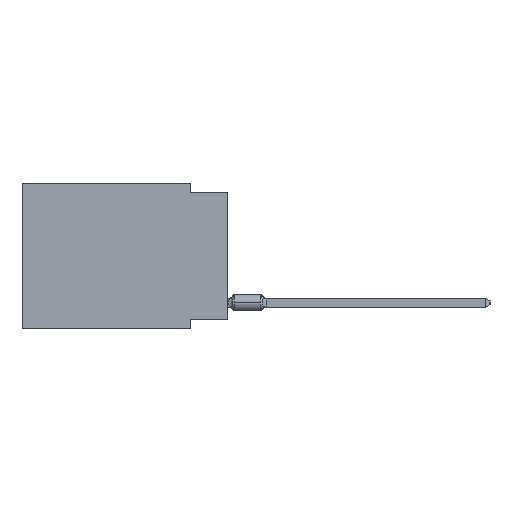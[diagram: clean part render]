
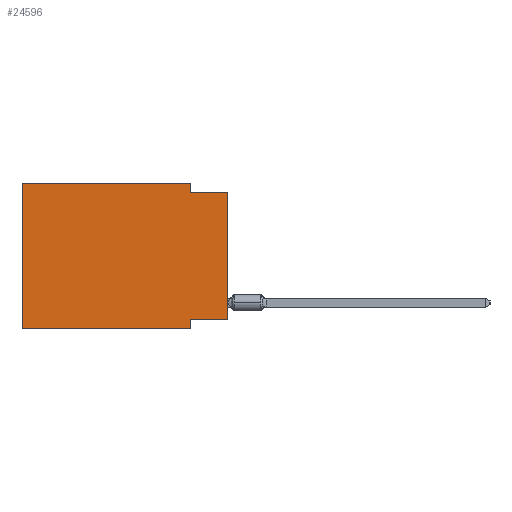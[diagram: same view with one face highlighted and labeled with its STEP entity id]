
A CAD part, left-side view. The second image highlights one B-rep face of the part: STEP entity #24596.
In plain terms, the highlighted planar face has unit normal (-1, 0, 0).
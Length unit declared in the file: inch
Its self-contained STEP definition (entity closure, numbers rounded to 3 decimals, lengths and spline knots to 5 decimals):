
#610 = VERTEX_POINT ( 'NONE', #2749 ) ;
#2749 = CARTESIAN_POINT ( 'NONE',  ( 0., 0., -0.365 ) ) ;
#4948 = CARTESIAN_POINT ( 'NONE',  ( 0., 0.1, -0.39 ) ) ;
#7659 = DIRECTION ( 'NONE',  ( 0., 0., -1. ) ) ;
#8100 = CARTESIAN_POINT ( 'NONE',  ( 0., 0.1, -0.365 ) ) ;
#8293 = VECTOR ( 'NONE', #47191, 39.37008 ) ;
#8863 = CARTESIAN_POINT ( 'NONE',  ( 0., 0.55, 0. ) ) ;
#9226 = EDGE_CURVE ( 'NONE', #38834, #43057, #32810, .T. ) ;
#9627 = CARTESIAN_POINT ( 'NONE',  ( 0., 0., 0. ) ) ;
#9933 = ORIENTED_EDGE ( 'NONE', *, *, #9226, .F. ) ;
#10651 = CARTESIAN_POINT ( 'NONE',  ( 0., 0.55, 0. ) ) ;
#10932 = ORIENTED_EDGE ( 'NONE', *, *, #39328, .T. ) ;
#12375 = CARTESIAN_POINT ( 'NONE',  ( 0., 0., -0.365 ) ) ;
#12977 = CARTESIAN_POINT ( 'NONE',  ( 0., 0.1, -0.39 ) ) ;
#13182 = ORIENTED_EDGE ( 'NONE', *, *, #44843, .F. ) ;
#13794 = CARTESIAN_POINT ( 'NONE',  ( 0., 0.55, -0.39 ) ) ;
#14665 = VECTOR ( 'NONE', #50113, 39.37008 ) ;
#14836 = EDGE_LOOP ( 'NONE', ( #10932, #9933, #33415, #44910, #13182, #35956, #22574, #25216 ) ) ;
#15957 = LINE ( 'NONE', #10651, #20593 ) ;
#17845 = VERTEX_POINT ( 'NONE', #8863 ) ;
#19046 = VECTOR ( 'NONE', #51093, 39.37008 ) ;
#19452 = DIRECTION ( 'NONE',  ( 0., 0., -1. ) ) ;
#20029 = EDGE_CURVE ( 'NONE', #17845, #27993, #15957, .T. ) ;
#20209 = CARTESIAN_POINT ( 'NONE',  ( 0., 0.1, 0. ) ) ;
#20593 = VECTOR ( 'NONE', #33013, 39.37008 ) ;
#22574 = ORIENTED_EDGE ( 'NONE', *, *, #30560, .F. ) ;
#23474 = AXIS2_PLACEMENT_3D ( 'NONE', #35681, #48251, #19452 ) ;
#24596 = ADVANCED_FACE ( 'NONE', ( #30937 ), #44902, .F. ) ;
#24976 = CARTESIAN_POINT ( 'NONE',  ( 0., 0.1, 0. ) ) ;
#25216 = ORIENTED_EDGE ( 'NONE', *, *, #45329, .F. ) ;
#25377 = LINE ( 'NONE', #42441, #19046 ) ;
#25840 = VERTEX_POINT ( 'NONE', #8100 ) ;
#26760 = CARTESIAN_POINT ( 'NONE',  ( 0., 0.1, -0.025 ) ) ;
#27993 = VERTEX_POINT ( 'NONE', #20209 ) ;
#28627 = LINE ( 'NONE', #24976, #43575 ) ;
#30213 = VECTOR ( 'NONE', #51909, 39.37008 ) ;
#30560 = EDGE_CURVE ( 'NONE', #25840, #35712, #34586, .T. ) ;
#30900 = LINE ( 'NONE', #9627, #38473 ) ;
#30937 = FACE_OUTER_BOUND ( 'NONE', #14836, .T. ) ;
#31711 = CARTESIAN_POINT ( 'NONE',  ( 0., 0., -0.025 ) ) ;
#32810 = LINE ( 'NONE', #31711, #50008 ) ;
#33013 = DIRECTION ( 'NONE',  ( 0., -1., 0. ) ) ;
#33415 = ORIENTED_EDGE ( 'NONE', *, *, #34367, .F. ) ;
#34330 = LINE ( 'NONE', #51377, #8293 ) ;
#34367 = EDGE_CURVE ( 'NONE', #27993, #38834, #28627, .T. ) ;
#34434 = VERTEX_POINT ( 'NONE', #13794 ) ;
#34586 = LINE ( 'NONE', #4948, #30213 ) ;
#35681 = CARTESIAN_POINT ( 'NONE',  ( 0., 0.55, 0. ) ) ;
#35712 = VERTEX_POINT ( 'NONE', #12977 ) ;
#35911 = DIRECTION ( 'NONE',  ( 0., 0., 1. ) ) ;
#35956 = ORIENTED_EDGE ( 'NONE', *, *, #47655, .T. ) ;
#38473 = VECTOR ( 'NONE', #35911, 39.37008 ) ;
#38834 = VERTEX_POINT ( 'NONE', #26760 ) ;
#39328 = EDGE_CURVE ( 'NONE', #610, #43057, #30900, .T. ) ;
#42441 = CARTESIAN_POINT ( 'NONE',  ( 0., 0.55, 0. ) ) ;
#43057 = VERTEX_POINT ( 'NONE', #46110 ) ;
#43575 = VECTOR ( 'NONE', #7659, 39.37008 ) ;
#44843 = EDGE_CURVE ( 'NONE', #34434, #17845, #25377, .T. ) ;
#44902 = PLANE ( 'NONE',  #23474 ) ;
#44910 = ORIENTED_EDGE ( 'NONE', *, *, #20029, .F. ) ;
#45329 = EDGE_CURVE ( 'NONE', #610, #25840, #55128, .T. ) ;
#46110 = CARTESIAN_POINT ( 'NONE',  ( 0., 0., -0.025 ) ) ;
#47191 = DIRECTION ( 'NONE',  ( 0., -1., 0. ) ) ;
#47655 = EDGE_CURVE ( 'NONE', #34434, #35712, #34330, .T. ) ;
#48251 = DIRECTION ( 'NONE',  ( 1., 0., 0. ) ) ;
#48754 = DIRECTION ( 'NONE',  ( 0., -1., 0. ) ) ;
#50008 = VECTOR ( 'NONE', #48754, 39.37008 ) ;
#50113 = DIRECTION ( 'NONE',  ( 0., 1., 0. ) ) ;
#51093 = DIRECTION ( 'NONE',  ( 0., 0., 1. ) ) ;
#51377 = CARTESIAN_POINT ( 'NONE',  ( 0., 0.55, -0.39 ) ) ;
#51909 = DIRECTION ( 'NONE',  ( 0., 0., -1. ) ) ;
#55128 = LINE ( 'NONE', #12375, #14665 ) ;
